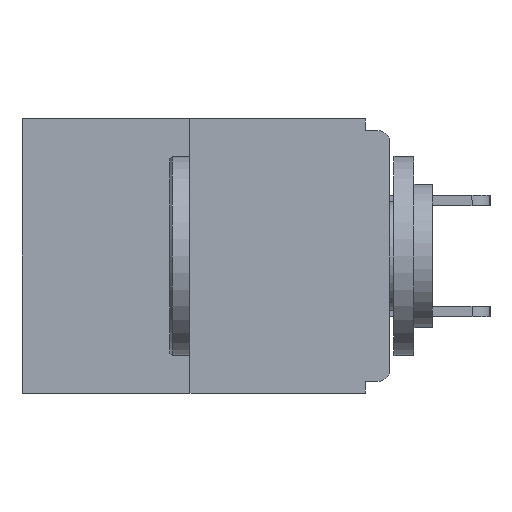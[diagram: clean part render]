
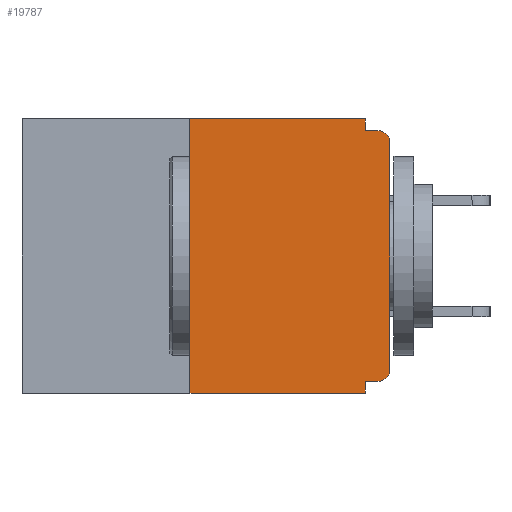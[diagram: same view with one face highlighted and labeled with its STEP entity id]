
A CAD part, left-side view. The second image highlights one B-rep face of the part: STEP entity #19787.
In plain terms, the highlighted planar face has unit normal (-1, 0, 0).
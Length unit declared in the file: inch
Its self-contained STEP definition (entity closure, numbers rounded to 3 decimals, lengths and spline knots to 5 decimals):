
#427 = EDGE_CURVE ( 'NONE', #13508, #11964, #14441, .T. ) ;
#507 = DIRECTION ( 'NONE',  ( 0., 0., -1. ) ) ;
#1237 = PLANE ( 'NONE',  #17826 ) ;
#1407 = LINE ( 'NONE', #5264, #9786 ) ;
#2055 = CARTESIAN_POINT ( 'NONE',  ( 0., 0., -0.03 ) ) ;
#2056 = DIRECTION ( 'NONE',  ( 0., 0., -1. ) ) ;
#2071 = VECTOR ( 'NONE', #19835, 39.37008 ) ;
#3055 = ORIENTED_EDGE ( 'NONE', *, *, #19657, .T. ) ;
#3230 = CARTESIAN_POINT ( 'NONE',  ( 0., 0.25, 0. ) ) ;
#3439 = VERTEX_POINT ( 'NONE', #6418 ) ;
#3902 = VECTOR ( 'NONE', #15304, 39.37008 ) ;
#3981 = EDGE_CURVE ( 'NONE', #10581, #12830, #18557, .T. ) ;
#4147 = CARTESIAN_POINT ( 'NONE',  ( 0., 0., 0. ) ) ;
#4335 = CARTESIAN_POINT ( 'NONE',  ( 0., 0.031, -0.015 ) ) ;
#4522 = ORIENTED_EDGE ( 'NONE', *, *, #12259, .F. ) ;
#4637 = EDGE_LOOP ( 'NONE', ( #27318, #4522, #14118, #11592, #7743, #10536, #27455, #3055, #19457, #22646 ) ) ;
#5264 = CARTESIAN_POINT ( 'NONE',  ( 0., 0.031, 0. ) ) ;
#5574 = DIRECTION ( 'NONE',  ( 0., 0., 1. ) ) ;
#5685 = CARTESIAN_POINT ( 'NONE',  ( 0., 0.46, 0. ) ) ;
#5921 = CIRCLE ( 'NONE', #27259, 0.015 ) ;
#5949 = CIRCLE ( 'NONE', #12346, 0.015 ) ;
#6418 = CARTESIAN_POINT ( 'NONE',  ( 0., 0.031, 0. ) ) ;
#6538 = CARTESIAN_POINT ( 'NONE',  ( 0., 0., -0.015 ) ) ;
#7463 = VERTEX_POINT ( 'NONE', #9679 ) ;
#7743 = ORIENTED_EDGE ( 'NONE', *, *, #17609, .F. ) ;
#7849 = CARTESIAN_POINT ( 'NONE',  ( 0., 0., -0.313 ) ) ;
#7969 = VECTOR ( 'NONE', #19931, 39.37008 ) ;
#8657 = CARTESIAN_POINT ( 'NONE',  ( 0., 0.031, -0.343 ) ) ;
#9163 = EDGE_CURVE ( 'NONE', #14784, #7463, #14747, .T. ) ;
#9251 = EDGE_CURVE ( 'NONE', #3439, #13508, #1407, .T. ) ;
#9679 = CARTESIAN_POINT ( 'NONE',  ( 0., 0.031, -0.343 ) ) ;
#9735 = CARTESIAN_POINT ( 'NONE',  ( 0., 0.015, -0.313 ) ) ;
#9786 = VECTOR ( 'NONE', #507, 39.37008 ) ;
#9950 = EDGE_CURVE ( 'NONE', #13032, #3439, #18564, .T. ) ;
#10051 = DIRECTION ( 'NONE',  ( 0., -1., 0. ) ) ;
#10536 = ORIENTED_EDGE ( 'NONE', *, *, #20185, .T. ) ;
#10581 = VERTEX_POINT ( 'NONE', #7849 ) ;
#11346 = VECTOR ( 'NONE', #16095, 39.37008 ) ;
#11592 = ORIENTED_EDGE ( 'NONE', *, *, #9163, .F. ) ;
#11709 = CARTESIAN_POINT ( 'NONE',  ( 0., 0.25, -0.343 ) ) ;
#11964 = VERTEX_POINT ( 'NONE', #15718 ) ;
#12181 = LINE ( 'NONE', #18711, #24853 ) ;
#12207 = VERTEX_POINT ( 'NONE', #16148 ) ;
#12232 = DIRECTION ( 'NONE',  ( 1., 0., 0. ) ) ;
#12259 = EDGE_CURVE ( 'NONE', #28580, #13032, #12181, .T. ) ;
#12346 = AXIS2_PLACEMENT_3D ( 'NONE', #24344, #22161, #2056 ) ;
#12830 = VERTEX_POINT ( 'NONE', #2055 ) ;
#12940 = VECTOR ( 'NONE', #10051, 39.37008 ) ;
#13032 = VERTEX_POINT ( 'NONE', #3230 ) ;
#13508 = VERTEX_POINT ( 'NONE', #4335 ) ;
#14118 = ORIENTED_EDGE ( 'NONE', *, *, #27074, .T. ) ;
#14441 = LINE ( 'NONE', #6538, #20757 ) ;
#14747 = LINE ( 'NONE', #8657, #3902 ) ;
#14784 = VERTEX_POINT ( 'NONE', #28087 ) ;
#14798 = CARTESIAN_POINT ( 'NONE',  ( 0., 0.46, 0. ) ) ;
#15304 = DIRECTION ( 'NONE',  ( 0., 0., -1. ) ) ;
#15718 = CARTESIAN_POINT ( 'NONE',  ( 0., 0.015, -0.015 ) ) ;
#16095 = DIRECTION ( 'NONE',  ( 0., 1., 0. ) ) ;
#16148 = CARTESIAN_POINT ( 'NONE',  ( 0., 0.015, -0.328 ) ) ;
#16437 = DIRECTION ( 'NONE',  ( 0., 0., -1. ) ) ;
#17609 = EDGE_CURVE ( 'NONE', #12207, #14784, #18385, .T. ) ;
#17826 = AXIS2_PLACEMENT_3D ( 'NONE', #5685, #12232, #18917 ) ;
#18385 = LINE ( 'NONE', #27315, #11346 ) ;
#18557 = LINE ( 'NONE', #4147, #2071 ) ;
#18564 = LINE ( 'NONE', #14798, #12940 ) ;
#18711 = CARTESIAN_POINT ( 'NONE',  ( 0., 0.25, 0. ) ) ;
#18917 = DIRECTION ( 'NONE',  ( 0., 0., -1. ) ) ;
#19457 = ORIENTED_EDGE ( 'NONE', *, *, #427, .F. ) ;
#19657 = EDGE_CURVE ( 'NONE', #12830, #11964, #5949, .T. ) ;
#19787 = ADVANCED_FACE ( 'NONE', ( #20005 ), #1237, .F. ) ;
#19835 = DIRECTION ( 'NONE',  ( 0., 0., 1. ) ) ;
#19931 = DIRECTION ( 'NONE',  ( 0., -1., 0. ) ) ;
#20005 = FACE_OUTER_BOUND ( 'NONE', #4637, .T. ) ;
#20185 = EDGE_CURVE ( 'NONE', #12207, #10581, #5921, .T. ) ;
#20757 = VECTOR ( 'NONE', #22351, 39.37008 ) ;
#20978 = DIRECTION ( 'NONE',  ( -1., 0., 0. ) ) ;
#22161 = DIRECTION ( 'NONE',  ( -1., 0., 0. ) ) ;
#22351 = DIRECTION ( 'NONE',  ( 0., -1., 0. ) ) ;
#22646 = ORIENTED_EDGE ( 'NONE', *, *, #9251, .F. ) ;
#24344 = CARTESIAN_POINT ( 'NONE',  ( 0., 0.015, -0.03 ) ) ;
#24653 = CARTESIAN_POINT ( 'NONE',  ( 0., 0.46, -0.343 ) ) ;
#24853 = VECTOR ( 'NONE', #5574, 39.37008 ) ;
#27074 = EDGE_CURVE ( 'NONE', #28580, #7463, #27347, .T. ) ;
#27259 = AXIS2_PLACEMENT_3D ( 'NONE', #9735, #20978, #16437 ) ;
#27315 = CARTESIAN_POINT ( 'NONE',  ( 0., 0., -0.328 ) ) ;
#27318 = ORIENTED_EDGE ( 'NONE', *, *, #9950, .F. ) ;
#27347 = LINE ( 'NONE', #24653, #7969 ) ;
#27455 = ORIENTED_EDGE ( 'NONE', *, *, #3981, .T. ) ;
#28087 = CARTESIAN_POINT ( 'NONE',  ( 0., 0.031, -0.328 ) ) ;
#28580 = VERTEX_POINT ( 'NONE', #11709 ) ;
